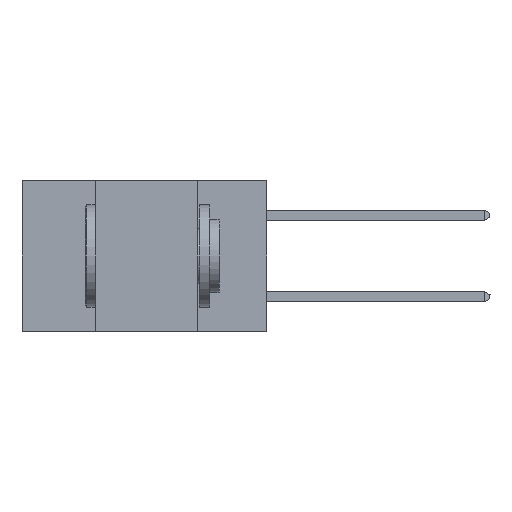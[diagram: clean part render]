
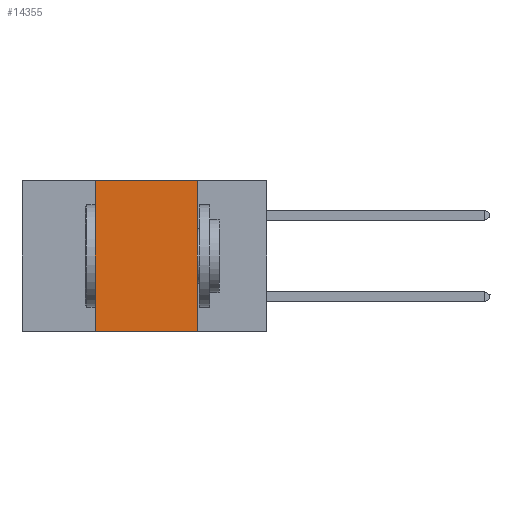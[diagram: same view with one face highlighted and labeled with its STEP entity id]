
A CAD part, left-side view. The second image highlights one B-rep face of the part: STEP entity #14355.
In plain terms, the highlighted planar face has unit normal (-1, 0, 0).
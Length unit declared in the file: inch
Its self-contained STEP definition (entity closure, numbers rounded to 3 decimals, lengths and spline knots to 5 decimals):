
#1085 = LINE ( 'NONE', #10463, #25408 ) ;
#3049 = CARTESIAN_POINT ( 'NONE',  ( 0., 0.42, 0. ) ) ;
#4576 = DIRECTION ( 'NONE',  ( 0., 0., -1. ) ) ;
#6778 = VERTEX_POINT ( 'NONE', #24227 ) ;
#7006 = ORIENTED_EDGE ( 'NONE', *, *, #25395, .F. ) ;
#7019 = EDGE_CURVE ( 'NONE', #27705, #6778, #10018, .T. ) ;
#9032 = DIRECTION ( 'NONE',  ( 0., -1., 0. ) ) ;
#10018 = LINE ( 'NONE', #12966, #25515 ) ;
#10221 = CARTESIAN_POINT ( 'NONE',  ( 0., 0.17, 0. ) ) ;
#10463 = CARTESIAN_POINT ( 'NONE',  ( 0., 0.6, -0.37 ) ) ;
#10959 = CARTESIAN_POINT ( 'NONE',  ( 0., 0.6, 0. ) ) ;
#11663 = CARTESIAN_POINT ( 'NONE',  ( 0., 0.42, -0.37 ) ) ;
#12413 = DIRECTION ( 'NONE',  ( 0., -1., 0. ) ) ;
#12966 = CARTESIAN_POINT ( 'NONE',  ( 0., 0.17, 0. ) ) ;
#13634 = ORIENTED_EDGE ( 'NONE', *, *, #7019, .F. ) ;
#14355 = ADVANCED_FACE ( 'NONE', ( #19039 ), #18260, .F. ) ;
#14772 = CARTESIAN_POINT ( 'NONE',  ( 0., 0.42, 0. ) ) ;
#14995 = AXIS2_PLACEMENT_3D ( 'NONE', #22598, #22406, #16089 ) ;
#15439 = VERTEX_POINT ( 'NONE', #11663 ) ;
#16089 = DIRECTION ( 'NONE',  ( 0., 0., -1. ) ) ;
#16241 = ORIENTED_EDGE ( 'NONE', *, *, #27286, .F. ) ;
#18260 = PLANE ( 'NONE',  #14995 ) ;
#19039 = FACE_OUTER_BOUND ( 'NONE', #24647, .T. ) ;
#20016 = VECTOR ( 'NONE', #27560, 39.37008 ) ;
#21714 = LINE ( 'NONE', #14772, #20016 ) ;
#21758 = EDGE_CURVE ( 'NONE', #15439, #6778, #1085, .T. ) ;
#21961 = LINE ( 'NONE', #10959, #25928 ) ;
#22406 = DIRECTION ( 'NONE',  ( 1., 0., 0. ) ) ;
#22598 = CARTESIAN_POINT ( 'NONE',  ( 0., 0.6, 0. ) ) ;
#23543 = VERTEX_POINT ( 'NONE', #3049 ) ;
#23634 = ORIENTED_EDGE ( 'NONE', *, *, #21758, .T. ) ;
#24227 = CARTESIAN_POINT ( 'NONE',  ( 0., 0.17, -0.37 ) ) ;
#24647 = EDGE_LOOP ( 'NONE', ( #13634, #16241, #7006, #23634 ) ) ;
#25395 = EDGE_CURVE ( 'NONE', #15439, #23543, #21714, .T. ) ;
#25408 = VECTOR ( 'NONE', #12413, 39.37008 ) ;
#25515 = VECTOR ( 'NONE', #4576, 39.37008 ) ;
#25928 = VECTOR ( 'NONE', #9032, 39.37008 ) ;
#27286 = EDGE_CURVE ( 'NONE', #23543, #27705, #21961, .T. ) ;
#27560 = DIRECTION ( 'NONE',  ( 0., 0., 1. ) ) ;
#27705 = VERTEX_POINT ( 'NONE', #10221 ) ;
